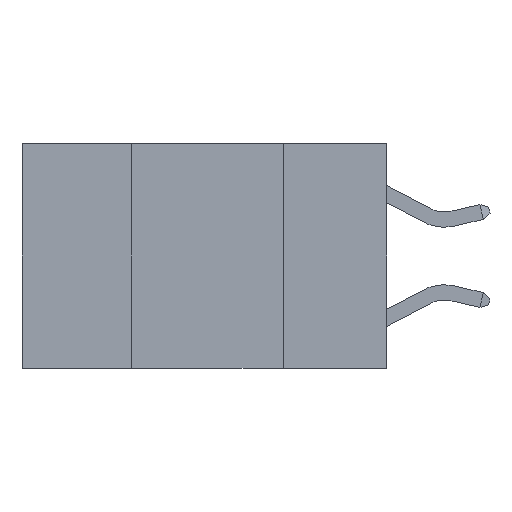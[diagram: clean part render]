
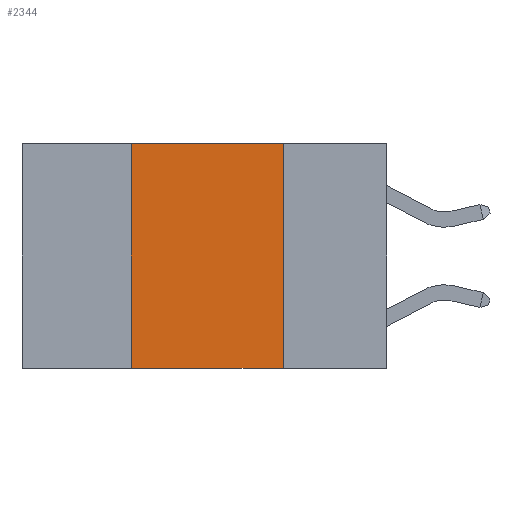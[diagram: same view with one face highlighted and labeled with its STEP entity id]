
A CAD part, left-side view. The second image highlights one B-rep face of the part: STEP entity #2344.
In plain terms, the highlighted planar face has unit normal (-1, 0, 0).
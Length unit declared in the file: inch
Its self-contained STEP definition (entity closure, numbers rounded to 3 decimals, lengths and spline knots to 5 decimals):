
#603 = PLANE ( 'NONE',  #4049 ) ;
#1093 = CARTESIAN_POINT ( 'NONE',  ( 0., 0.17, 0. ) ) ;
#1293 = EDGE_CURVE ( 'NONE', #6823, #8399, #3534, .T. ) ;
#1397 = ORIENTED_EDGE ( 'NONE', *, *, #6740, .F. ) ;
#2344 = ADVANCED_FACE ( 'NONE', ( #6607 ), #603, .F. ) ;
#3063 = DIRECTION ( 'NONE',  ( 1., 0., 0. ) ) ;
#3186 = DIRECTION ( 'NONE',  ( 0., -1., 0. ) ) ;
#3534 = LINE ( 'NONE', #9707, #5387 ) ;
#3991 = CARTESIAN_POINT ( 'NONE',  ( 0., 0.42, -0.37 ) ) ;
#4035 = LINE ( 'NONE', #1093, #9914 ) ;
#4049 = AXIS2_PLACEMENT_3D ( 'NONE', #4632, #3063, #8612 ) ;
#4305 = EDGE_CURVE ( 'NONE', #7802, #8399, #4035, .T. ) ;
#4437 = ORIENTED_EDGE ( 'NONE', *, *, #1293, .T. ) ;
#4620 = VECTOR ( 'NONE', #10255, 39.37008 ) ;
#4632 = CARTESIAN_POINT ( 'NONE',  ( 0., 0.6, 0. ) ) ;
#4811 = CARTESIAN_POINT ( 'NONE',  ( 0., 0.6, 0. ) ) ;
#5387 = VECTOR ( 'NONE', #7314, 39.37008 ) ;
#5896 = EDGE_CURVE ( 'NONE', #7049, #7802, #5994, .T. ) ;
#5994 = LINE ( 'NONE', #4811, #6222 ) ;
#6046 = ORIENTED_EDGE ( 'NONE', *, *, #4305, .F. ) ;
#6222 = VECTOR ( 'NONE', #3186, 39.37008 ) ;
#6607 = FACE_OUTER_BOUND ( 'NONE', #7869, .T. ) ;
#6740 = EDGE_CURVE ( 'NONE', #6823, #7049, #7218, .T. ) ;
#6823 = VERTEX_POINT ( 'NONE', #3991 ) ;
#7049 = VERTEX_POINT ( 'NONE', #9028 ) ;
#7218 = LINE ( 'NONE', #9468, #4620 ) ;
#7314 = DIRECTION ( 'NONE',  ( 0., -1., 0. ) ) ;
#7480 = DIRECTION ( 'NONE',  ( 0., 0., -1. ) ) ;
#7558 = CARTESIAN_POINT ( 'NONE',  ( 0., 0.17, 0. ) ) ;
#7802 = VERTEX_POINT ( 'NONE', #7558 ) ;
#7869 = EDGE_LOOP ( 'NONE', ( #6046, #9527, #1397, #4437 ) ) ;
#8399 = VERTEX_POINT ( 'NONE', #8419 ) ;
#8419 = CARTESIAN_POINT ( 'NONE',  ( 0., 0.17, -0.37 ) ) ;
#8612 = DIRECTION ( 'NONE',  ( 0., 0., -1. ) ) ;
#9028 = CARTESIAN_POINT ( 'NONE',  ( 0., 0.42, 0. ) ) ;
#9468 = CARTESIAN_POINT ( 'NONE',  ( 0., 0.42, 0. ) ) ;
#9527 = ORIENTED_EDGE ( 'NONE', *, *, #5896, .F. ) ;
#9707 = CARTESIAN_POINT ( 'NONE',  ( 0., 0.6, -0.37 ) ) ;
#9914 = VECTOR ( 'NONE', #7480, 39.37008 ) ;
#10255 = DIRECTION ( 'NONE',  ( 0., 0., 1. ) ) ;
